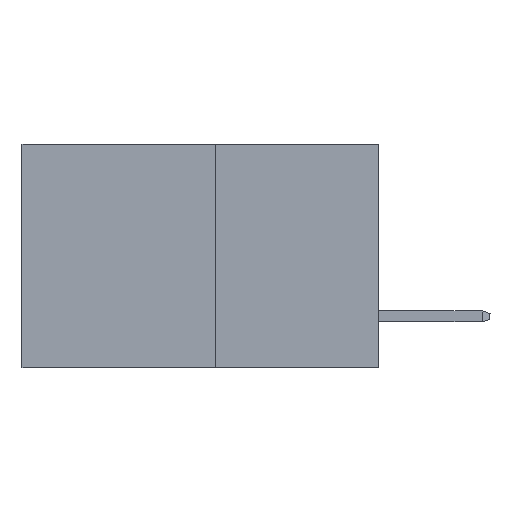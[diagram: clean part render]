
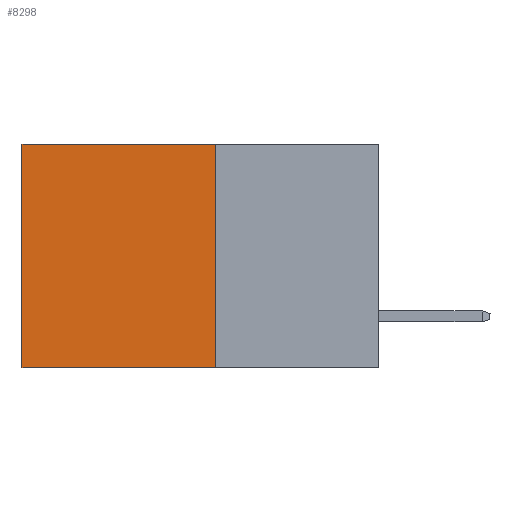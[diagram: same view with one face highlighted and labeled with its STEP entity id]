
A CAD part, left-side view. The second image highlights one B-rep face of the part: STEP entity #8298.
In plain terms, the highlighted planar face has unit normal (-1, 0, 0).
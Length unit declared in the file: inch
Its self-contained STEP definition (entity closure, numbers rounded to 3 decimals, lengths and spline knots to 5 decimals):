
#78 = LINE ( 'NONE', #7383, #5916 ) ;
#171 = LINE ( 'NONE', #6015, #4330 ) ;
#172 = CARTESIAN_POINT ( 'NONE',  ( 0.277, 0.27, -0.37 ) ) ;
#242 = LINE ( 'NONE', #5469, #2114 ) ;
#1220 = CARTESIAN_POINT ( 'NONE',  ( 0.277, 0.59, 0. ) ) ;
#1601 = EDGE_LOOP ( 'NONE', ( #2598, #3930, #4304, #5288 ) ) ;
#1730 = CARTESIAN_POINT ( 'NONE',  ( 0.277, 0.27, -0.37 ) ) ;
#1817 = VERTEX_POINT ( 'NONE', #2658 ) ;
#2114 = VECTOR ( 'NONE', #6312, 39.37008 ) ;
#2384 = CARTESIAN_POINT ( 'NONE',  ( 0.277, 0.59, -0.37 ) ) ;
#2402 = DIRECTION ( 'NONE',  ( 0., 0., -1. ) ) ;
#2486 = DIRECTION ( 'NONE',  ( 0., 0., -1. ) ) ;
#2598 = ORIENTED_EDGE ( 'NONE', *, *, #6519, .T. ) ;
#2658 = CARTESIAN_POINT ( 'NONE',  ( 0.277, 0.59, -0.37 ) ) ;
#2784 = EDGE_CURVE ( 'NONE', #3553, #3157, #242, .T. ) ;
#3157 = VERTEX_POINT ( 'NONE', #1220 ) ;
#3553 = VERTEX_POINT ( 'NONE', #6195 ) ;
#3855 = FACE_OUTER_BOUND ( 'NONE', #1601, .T. ) ;
#3930 = ORIENTED_EDGE ( 'NONE', *, *, #6323, .F. ) ;
#4304 = ORIENTED_EDGE ( 'NONE', *, *, #4756, .F. ) ;
#4330 = VECTOR ( 'NONE', #5976, 39.37008 ) ;
#4457 = VECTOR ( 'NONE', #2402, 39.37008 ) ;
#4756 = EDGE_CURVE ( 'NONE', #3553, #8337, #78, .T. ) ;
#5288 = ORIENTED_EDGE ( 'NONE', *, *, #2784, .T. ) ;
#5469 = CARTESIAN_POINT ( 'NONE',  ( 0.277, 0.27, 0. ) ) ;
#5916 = VECTOR ( 'NONE', #7398, 39.37008 ) ;
#5976 = DIRECTION ( 'NONE',  ( 0., 1., 0. ) ) ;
#6015 = CARTESIAN_POINT ( 'NONE',  ( 0.277, 0.27, -0.37 ) ) ;
#6171 = PLANE ( 'NONE',  #6361 ) ;
#6195 = CARTESIAN_POINT ( 'NONE',  ( 0.277, 0.27, 0. ) ) ;
#6312 = DIRECTION ( 'NONE',  ( 0., 1., 0. ) ) ;
#6323 = EDGE_CURVE ( 'NONE', #8337, #1817, #171, .T. ) ;
#6361 = AXIS2_PLACEMENT_3D ( 'NONE', #1730, #6889, #2486 ) ;
#6519 = EDGE_CURVE ( 'NONE', #3157, #1817, #8239, .T. ) ;
#6889 = DIRECTION ( 'NONE',  ( 1., 0., 0. ) ) ;
#7383 = CARTESIAN_POINT ( 'NONE',  ( 0.277, 0.27, -0.37 ) ) ;
#7398 = DIRECTION ( 'NONE',  ( 0., 0., -1. ) ) ;
#8239 = LINE ( 'NONE', #2384, #4457 ) ;
#8298 = ADVANCED_FACE ( 'NONE', ( #3855 ), #6171, .F. ) ;
#8337 = VERTEX_POINT ( 'NONE', #172 ) ;
